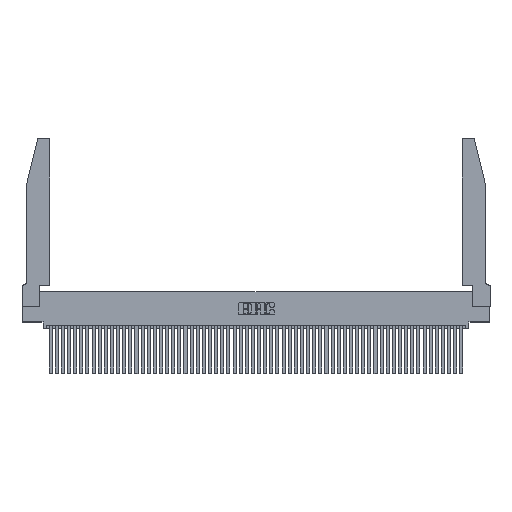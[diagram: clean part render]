
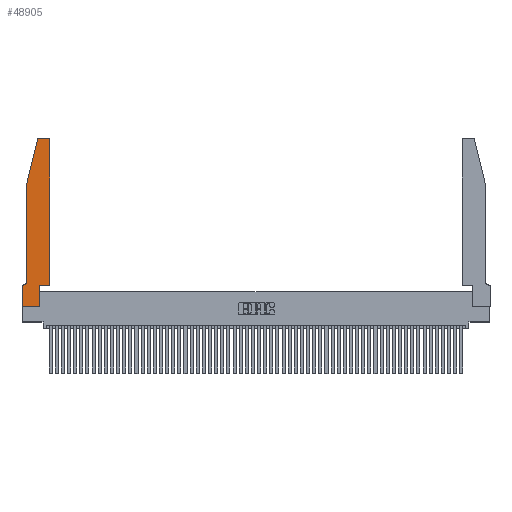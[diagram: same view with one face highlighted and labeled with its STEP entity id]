
A CAD part, top view. The second image highlights one B-rep face of the part: STEP entity #48905.
In plain terms, the highlighted planar face has unit normal (0, 0, 1).
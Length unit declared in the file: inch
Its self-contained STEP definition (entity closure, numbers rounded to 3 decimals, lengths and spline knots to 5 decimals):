
#1003 = VERTEX_POINT ( 'NONE', #48353 ) ;
#1214 = CARTESIAN_POINT ( 'NONE',  ( 0.0055, 0.42, 0.37 ) ) ;
#2320 = ORIENTED_EDGE ( 'NONE', *, *, #38479, .T. ) ;
#3922 = AXIS2_PLACEMENT_3D ( 'NONE', #1214, #22512, #43382 ) ;
#4909 = EDGE_CURVE ( 'NONE', #12145, #43317, #44018, .T. ) ;
#5089 = CARTESIAN_POINT ( 'NONE',  ( 0.284, 2.75, 0.37 ) ) ;
#6069 = EDGE_CURVE ( 'NONE', #1003, #15843, #54465, .T. ) ;
#6256 = DIRECTION ( 'NONE',  ( 0., -1., 0. ) ) ;
#6481 = CARTESIAN_POINT ( 'NONE',  ( 0., 0., 0.37 ) ) ;
#6539 = VERTEX_POINT ( 'NONE', #21984 ) ;
#8226 = DIRECTION ( 'NONE',  ( 1., 0., 0. ) ) ;
#9017 = CARTESIAN_POINT ( 'NONE',  ( 0.2605, 2.75, 0.37 ) ) ;
#9262 = LINE ( 'NONE', #13608, #32324 ) ;
#9329 = EDGE_CURVE ( 'NONE', #21640, #25483, #52082, .T. ) ;
#10024 = CARTESIAN_POINT ( 'NONE',  ( 0.4505, 0.35, 0.37 ) ) ;
#10208 = DIRECTION ( 'NONE',  ( 0., 1., 0. ) ) ;
#10659 = DIRECTION ( 'NONE',  ( 1., 0., 0. ) ) ;
#11331 = LINE ( 'NONE', #35206, #29833 ) ;
#11384 = VERTEX_POINT ( 'NONE', #16190 ) ;
#12145 = VERTEX_POINT ( 'NONE', #45995 ) ;
#12773 = CIRCLE ( 'NONE', #33650, 0.03 ) ;
#13111 = CARTESIAN_POINT ( 'NONE',  ( 0.0755, 0.35, 0.37 ) ) ;
#13608 = CARTESIAN_POINT ( 'NONE',  ( 0.2865, 0.35, 0.37 ) ) ;
#13745 = ORIENTED_EDGE ( 'NONE', *, *, #9329, .T. ) ;
#13878 = DIRECTION ( 'NONE',  ( 0., 0., 1. ) ) ;
#14672 = EDGE_CURVE ( 'NONE', #54090, #34448, #21870, .T. ) ;
#14740 = CARTESIAN_POINT ( 'NONE',  ( 0.4205, 2.75, 0.37 ) ) ;
#15072 = LINE ( 'NONE', #9017, #52108 ) ;
#15129 = CARTESIAN_POINT ( 'NONE',  ( 0., 0., 0.37 ) ) ;
#15191 = VECTOR ( 'NONE', #46263, 39.37008 ) ;
#15336 = EDGE_CURVE ( 'NONE', #6539, #1003, #9262, .T. ) ;
#15843 = VERTEX_POINT ( 'NONE', #17652 ) ;
#16190 = CARTESIAN_POINT ( 'NONE',  ( 0.25487, 2.72718, 0.37 ) ) ;
#16546 = VECTOR ( 'NONE', #42650, 39.37008 ) ;
#17236 = ORIENTED_EDGE ( 'NONE', *, *, #33346, .T. ) ;
#17652 = CARTESIAN_POINT ( 'NONE',  ( 0.4505, 0.35, 0.37 ) ) ;
#17761 = VECTOR ( 'NONE', #6256, 39.37008 ) ;
#18276 = FACE_OUTER_BOUND ( 'NONE', #19635, .T. ) ;
#18485 = DIRECTION ( 'NONE',  ( 1., 0., 0. ) ) ;
#19635 = EDGE_LOOP ( 'NONE', ( #34821, #24834, #2320, #17236, #25126, #44871, #13745, #21541, #54226, #20781, #28653, #26279 ) ) ;
#20112 = EDGE_CURVE ( 'NONE', #15843, #12145, #21471, .T. ) ;
#20781 = ORIENTED_EDGE ( 'NONE', *, *, #6069, .T. ) ;
#21471 = LINE ( 'NONE', #10024, #37310 ) ;
#21541 = ORIENTED_EDGE ( 'NONE', *, *, #22389, .T. ) ;
#21640 = VERTEX_POINT ( 'NONE', #23734 ) ;
#21870 = CIRCLE ( 'NONE', #3922, 0.07 ) ;
#21984 = CARTESIAN_POINT ( 'NONE',  ( 0.2865, 0., 0.37 ) ) ;
#22389 = EDGE_CURVE ( 'NONE', #25483, #6539, #22634, .T. ) ;
#22512 = DIRECTION ( 'NONE',  ( 0., 0., -1. ) ) ;
#22634 = LINE ( 'NONE', #6481, #29278 ) ;
#23734 = CARTESIAN_POINT ( 'NONE',  ( 0., 0.35, 0.37 ) ) ;
#24640 = EDGE_CURVE ( 'NONE', #43317, #47209, #15072, .T. ) ;
#24834 = ORIENTED_EDGE ( 'NONE', *, *, #46188, .T. ) ;
#25013 = CARTESIAN_POINT ( 'NONE',  ( 0.4205, 2.72, 0.37 ) ) ;
#25126 = ORIENTED_EDGE ( 'NONE', *, *, #14672, .T. ) ;
#25454 = CARTESIAN_POINT ( 'NONE',  ( 0.4505, 0.35, 0.37 ) ) ;
#25483 = VERTEX_POINT ( 'NONE', #15129 ) ;
#25808 = CARTESIAN_POINT ( 'NONE',  ( 0.0755, 2., 0.37 ) ) ;
#26279 = ORIENTED_EDGE ( 'NONE', *, *, #4909, .T. ) ;
#26406 = DIRECTION ( 'NONE',  ( 1., 0., 0. ) ) ;
#27727 = CARTESIAN_POINT ( 'NONE',  ( 0.0055, 0.35, 0.37 ) ) ;
#27757 = LINE ( 'NONE', #25808, #15191 ) ;
#28653 = ORIENTED_EDGE ( 'NONE', *, *, #20112, .T. ) ;
#29278 = VECTOR ( 'NONE', #10659, 39.37008 ) ;
#29833 = VECTOR ( 'NONE', #43703, 39.37008 ) ;
#30782 = DIRECTION ( 'NONE',  ( 0., 1., 0. ) ) ;
#31483 = CARTESIAN_POINT ( 'NONE',  ( 0., 0., 0.37 ) ) ;
#31512 = VERTEX_POINT ( 'NONE', #44576 ) ;
#32324 = VECTOR ( 'NONE', #30782, 39.37008 ) ;
#33346 = EDGE_CURVE ( 'NONE', #31512, #54090, #27757, .T. ) ;
#33466 = DIRECTION ( 'NONE',  ( 0., 0., 1. ) ) ;
#33650 = AXIS2_PLACEMENT_3D ( 'NONE', #39180, #13878, #18485 ) ;
#33715 = DIRECTION ( 'NONE',  ( 1., 0., 0. ) ) ;
#34448 = VERTEX_POINT ( 'NONE', #27727 ) ;
#34685 = PLANE ( 'NONE',  #53888 ) ;
#34821 = ORIENTED_EDGE ( 'NONE', *, *, #24640, .T. ) ;
#35048 = LINE ( 'NONE', #13111, #16546 ) ;
#35206 = CARTESIAN_POINT ( 'NONE',  ( 0.0755, 2., 0.37 ) ) ;
#37310 = VECTOR ( 'NONE', #10208, 39.37008 ) ;
#38479 = EDGE_CURVE ( 'NONE', #11384, #31512, #11331, .T. ) ;
#39180 = CARTESIAN_POINT ( 'NONE',  ( 0.284, 2.72, 0.37 ) ) ;
#42650 = DIRECTION ( 'NONE',  ( -1., 0., 0. ) ) ;
#43237 = VECTOR ( 'NONE', #33715, 39.37008 ) ;
#43317 = VERTEX_POINT ( 'NONE', #14740 ) ;
#43319 = CARTESIAN_POINT ( 'NONE',  ( 0.0755, 0.42, 0.37 ) ) ;
#43382 = DIRECTION ( 'NONE',  ( -1., 0., 0. ) ) ;
#43703 = DIRECTION ( 'NONE',  ( -0.239, -0.971, 0. ) ) ;
#44018 = CIRCLE ( 'NONE', #52342, 0.03 ) ;
#44576 = CARTESIAN_POINT ( 'NONE',  ( 0.0755, 2., 0.37 ) ) ;
#44871 = ORIENTED_EDGE ( 'NONE', *, *, #53253, .T. ) ;
#45995 = CARTESIAN_POINT ( 'NONE',  ( 0.4505, 2.72, 0.37 ) ) ;
#46188 = EDGE_CURVE ( 'NONE', #47209, #11384, #12773, .T. ) ;
#46263 = DIRECTION ( 'NONE',  ( 0., -1., 0. ) ) ;
#47209 = VERTEX_POINT ( 'NONE', #5089 ) ;
#48353 = CARTESIAN_POINT ( 'NONE',  ( 0.2865, 0.35, 0.37 ) ) ;
#48905 = ADVANCED_FACE ( 'NONE', ( #18276 ), #34685, .T. ) ;
#51276 = DIRECTION ( 'NONE',  ( -1., 0., 0. ) ) ;
#51328 = CARTESIAN_POINT ( 'NONE',  ( 0., 0.35, 0.37 ) ) ;
#52045 = DIRECTION ( 'NONE',  ( 0., 0., 1. ) ) ;
#52082 = LINE ( 'NONE', #31483, #17761 ) ;
#52108 = VECTOR ( 'NONE', #51276, 39.37008 ) ;
#52342 = AXIS2_PLACEMENT_3D ( 'NONE', #25013, #33466, #8226 ) ;
#53253 = EDGE_CURVE ( 'NONE', #34448, #21640, #35048, .T. ) ;
#53888 = AXIS2_PLACEMENT_3D ( 'NONE', #51328, #52045, #26406 ) ;
#54090 = VERTEX_POINT ( 'NONE', #43319 ) ;
#54226 = ORIENTED_EDGE ( 'NONE', *, *, #15336, .T. ) ;
#54465 = LINE ( 'NONE', #25454, #43237 ) ;
